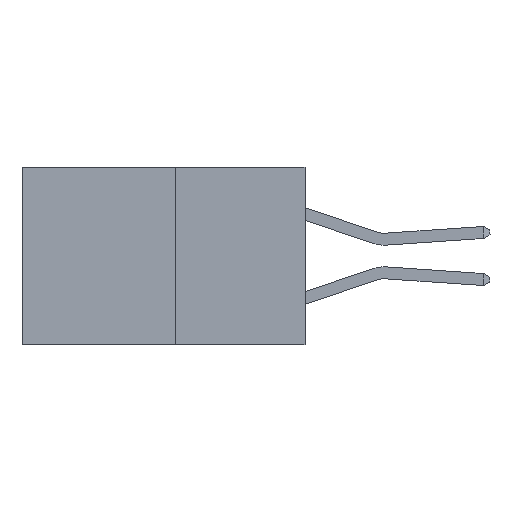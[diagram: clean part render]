
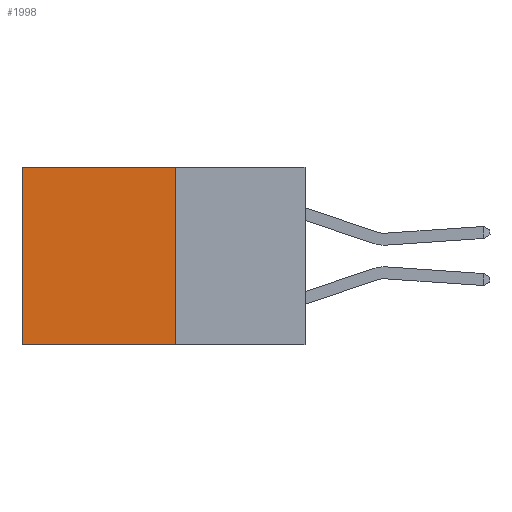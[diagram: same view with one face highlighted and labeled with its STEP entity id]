
A CAD part, left-side view. The second image highlights one B-rep face of the part: STEP entity #1998.
In plain terms, the highlighted planar face has unit normal (-1, 0, 0).
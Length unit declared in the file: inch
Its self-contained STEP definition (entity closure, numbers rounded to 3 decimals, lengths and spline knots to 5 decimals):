
#64 = CARTESIAN_POINT ( 'NONE',  ( 0.277, 0.27, -0.37 ) ) ;
#436 = DIRECTION ( 'NONE',  ( 0., 1., 0. ) ) ;
#877 = CARTESIAN_POINT ( 'NONE',  ( 0.277, 0.27, -0.37 ) ) ;
#908 = ORIENTED_EDGE ( 'NONE', *, *, #3403, .T. ) ;
#1235 = LINE ( 'NONE', #10629, #8198 ) ;
#1833 = CARTESIAN_POINT ( 'NONE',  ( 0.277, 0.27, -0.37 ) ) ;
#1962 = EDGE_LOOP ( 'NONE', ( #7694, #10407, #8119, #908 ) ) ;
#1965 = PLANE ( 'NONE',  #2250 ) ;
#1998 = ADVANCED_FACE ( 'NONE', ( #2697 ), #1965, .F. ) ;
#2250 = AXIS2_PLACEMENT_3D ( 'NONE', #877, #9698, #10347 ) ;
#2697 = FACE_OUTER_BOUND ( 'NONE', #1962, .T. ) ;
#2710 = VERTEX_POINT ( 'NONE', #1833 ) ;
#3403 = EDGE_CURVE ( 'NONE', #9615, #6677, #1235, .T. ) ;
#4524 = CARTESIAN_POINT ( 'NONE',  ( 0.277, 0.27, -0.37 ) ) ;
#4742 = DIRECTION ( 'NONE',  ( 0., 0., -1. ) ) ;
#4862 = DIRECTION ( 'NONE',  ( 0., 1., 0. ) ) ;
#4992 = EDGE_CURVE ( 'NONE', #6677, #9355, #6459, .T. ) ;
#5450 = EDGE_CURVE ( 'NONE', #2710, #9355, #8832, .T. ) ;
#6141 = CARTESIAN_POINT ( 'NONE',  ( 0.277, 0.59, -0.37 ) ) ;
#6459 = LINE ( 'NONE', #7098, #10842 ) ;
#6677 = VERTEX_POINT ( 'NONE', #10922 ) ;
#7098 = CARTESIAN_POINT ( 'NONE',  ( 0.277, 0.59, -0.37 ) ) ;
#7694 = ORIENTED_EDGE ( 'NONE', *, *, #4992, .T. ) ;
#7824 = VECTOR ( 'NONE', #4742, 39.37008 ) ;
#8111 = LINE ( 'NONE', #64, #7824 ) ;
#8119 = ORIENTED_EDGE ( 'NONE', *, *, #10256, .F. ) ;
#8198 = VECTOR ( 'NONE', #436, 39.37008 ) ;
#8832 = LINE ( 'NONE', #4524, #10832 ) ;
#9167 = CARTESIAN_POINT ( 'NONE',  ( 0.277, 0.27, 0. ) ) ;
#9355 = VERTEX_POINT ( 'NONE', #6141 ) ;
#9615 = VERTEX_POINT ( 'NONE', #9167 ) ;
#9698 = DIRECTION ( 'NONE',  ( 1., 0., 0. ) ) ;
#10015 = DIRECTION ( 'NONE',  ( 0., 0., -1. ) ) ;
#10256 = EDGE_CURVE ( 'NONE', #9615, #2710, #8111, .T. ) ;
#10347 = DIRECTION ( 'NONE',  ( 0., 0., -1. ) ) ;
#10407 = ORIENTED_EDGE ( 'NONE', *, *, #5450, .F. ) ;
#10629 = CARTESIAN_POINT ( 'NONE',  ( 0.277, 0.27, 0. ) ) ;
#10832 = VECTOR ( 'NONE', #4862, 39.37008 ) ;
#10842 = VECTOR ( 'NONE', #10015, 39.37008 ) ;
#10922 = CARTESIAN_POINT ( 'NONE',  ( 0.277, 0.59, 0. ) ) ;
